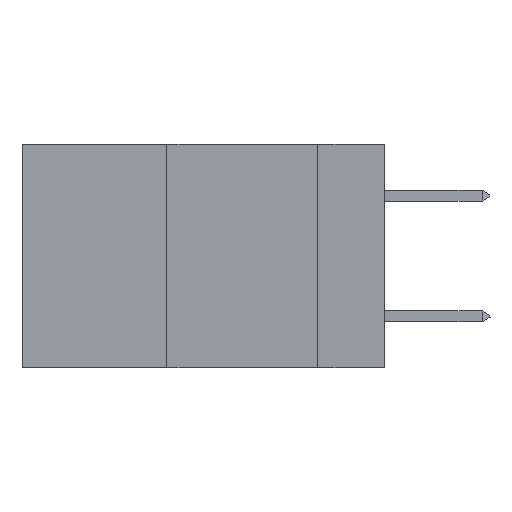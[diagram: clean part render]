
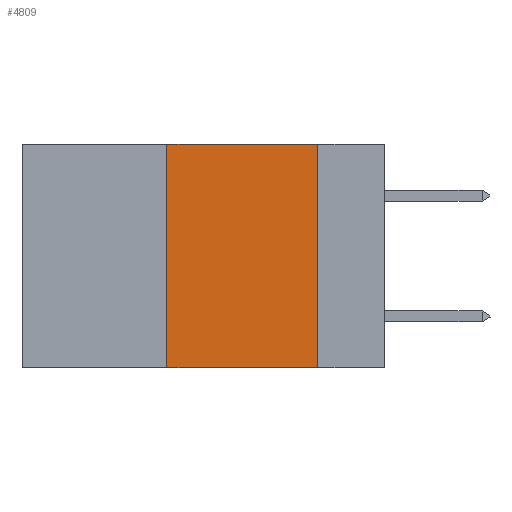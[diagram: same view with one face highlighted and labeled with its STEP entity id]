
A CAD part, left-side view. The second image highlights one B-rep face of the part: STEP entity #4809.
In plain terms, the highlighted planar face has unit normal (-1, 0, 0).
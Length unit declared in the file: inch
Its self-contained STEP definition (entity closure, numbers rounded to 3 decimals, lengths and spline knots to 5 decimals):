
#90 = CARTESIAN_POINT ( 'NONE',  ( 0., 0.36, 0. ) ) ;
#601 = VERTEX_POINT ( 'NONE', #1794 ) ;
#1287 = ORIENTED_EDGE ( 'NONE', *, *, #4268, .F. ) ;
#1367 = EDGE_CURVE ( 'NONE', #3577, #601, #10318, .T. ) ;
#1794 = CARTESIAN_POINT ( 'NONE',  ( 0., 0.11, -0.37 ) ) ;
#2626 = VECTOR ( 'NONE', #8539, 39.37008 ) ;
#2637 = LINE ( 'NONE', #8247, #5495 ) ;
#3079 = DIRECTION ( 'NONE',  ( 0., 0., -1. ) ) ;
#3544 = VECTOR ( 'NONE', #3079, 39.37008 ) ;
#3553 = CARTESIAN_POINT ( 'NONE',  ( 0., 0.11, 0. ) ) ;
#3577 = VERTEX_POINT ( 'NONE', #3946 ) ;
#3632 = DIRECTION ( 'NONE',  ( 0., -1., 0. ) ) ;
#3946 = CARTESIAN_POINT ( 'NONE',  ( 0., 0.36, -0.37 ) ) ;
#3991 = LINE ( 'NONE', #8745, #3544 ) ;
#4115 = ORIENTED_EDGE ( 'NONE', *, *, #1367, .T. ) ;
#4268 = EDGE_CURVE ( 'NONE', #3577, #6342, #5190, .T. ) ;
#4684 = CARTESIAN_POINT ( 'NONE',  ( 0., 0.6, -0.37 ) ) ;
#4762 = CARTESIAN_POINT ( 'NONE',  ( 0., 0.36, 0. ) ) ;
#4809 = ADVANCED_FACE ( 'NONE', ( #12356 ), #5488, .F. ) ;
#5103 = VECTOR ( 'NONE', #8472, 39.37008 ) ;
#5190 = LINE ( 'NONE', #4762, #2626 ) ;
#5488 = PLANE ( 'NONE',  #9406 ) ;
#5495 = VECTOR ( 'NONE', #3632, 39.37008 ) ;
#5875 = ORIENTED_EDGE ( 'NONE', *, *, #6942, .F. ) ;
#6342 = VERTEX_POINT ( 'NONE', #90 ) ;
#6485 = DIRECTION ( 'NONE',  ( 1., 0., 0. ) ) ;
#6726 = ORIENTED_EDGE ( 'NONE', *, *, #7271, .F. ) ;
#6892 = VERTEX_POINT ( 'NONE', #3553 ) ;
#6942 = EDGE_CURVE ( 'NONE', #6342, #6892, #2637, .T. ) ;
#7271 = EDGE_CURVE ( 'NONE', #6892, #601, #3991, .T. ) ;
#8247 = CARTESIAN_POINT ( 'NONE',  ( 0., 0.6, 0. ) ) ;
#8472 = DIRECTION ( 'NONE',  ( 0., -1., 0. ) ) ;
#8539 = DIRECTION ( 'NONE',  ( 0., 0., 1. ) ) ;
#8745 = CARTESIAN_POINT ( 'NONE',  ( 0., 0.11, 0. ) ) ;
#9406 = AXIS2_PLACEMENT_3D ( 'NONE', #12193, #6485, #10359 ) ;
#10318 = LINE ( 'NONE', #4684, #5103 ) ;
#10359 = DIRECTION ( 'NONE',  ( 0., 0., -1. ) ) ;
#10699 = EDGE_LOOP ( 'NONE', ( #6726, #5875, #1287, #4115 ) ) ;
#12193 = CARTESIAN_POINT ( 'NONE',  ( 0., 0.6, 0. ) ) ;
#12356 = FACE_OUTER_BOUND ( 'NONE', #10699, .T. ) ;
